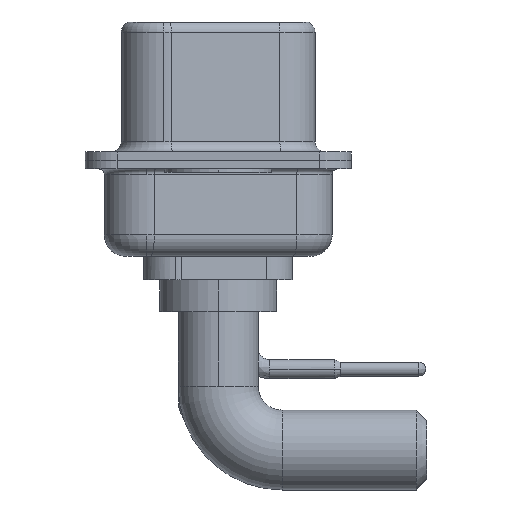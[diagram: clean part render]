
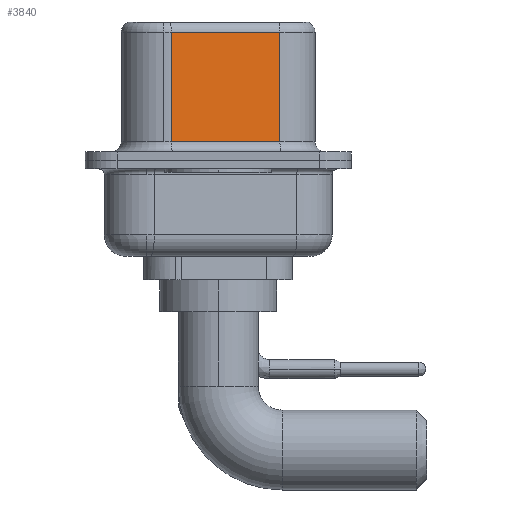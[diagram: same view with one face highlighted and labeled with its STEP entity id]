
A CAD part, left-side view. The second image highlights one B-rep face of the part: STEP entity #3840.
In plain terms, the highlighted planar face has unit normal (-0.985, -0.174, 0).
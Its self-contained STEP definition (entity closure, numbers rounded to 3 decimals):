
#580 = FACE_OUTER_BOUND ( 'NONE', #864, .T. ) ;
#864 = EDGE_LOOP ( 'NONE', ( #958, #6412, #3477, #17819 ) ) ;
#927 = EDGE_CURVE ( 'NONE', #14997, #15901, #13058, .T. ) ;
#958 = ORIENTED_EDGE ( 'NONE', *, *, #11378, .F. ) ;
#1845 = CARTESIAN_POINT ( 'NONE',  ( 4.555, -2.897, 0.9 ) ) ;
#2016 = DIRECTION ( 'NONE',  ( 0.985, 0.174, 0. ) ) ;
#2965 = CARTESIAN_POINT ( 'NONE',  ( 3.655, 2.203, 0.9 ) ) ;
#3426 = VECTOR ( 'NONE', #6063, 1000. ) ;
#3477 = ORIENTED_EDGE ( 'NONE', *, *, #8779, .T. ) ;
#3755 = DIRECTION ( 'NONE',  ( -0.174, 0.985, 0. ) ) ;
#3840 = ADVANCED_FACE ( 'NONE', ( #580 ), #7730, .F. ) ;
#4393 = VECTOR ( 'NONE', #17461, 1000. ) ;
#4451 = VECTOR ( 'NONE', #6938, 1000. ) ;
#4848 = VERTEX_POINT ( 'NONE', #15828 ) ;
#6063 = DIRECTION ( 'NONE',  ( 0., 0., -1. ) ) ;
#6412 = ORIENTED_EDGE ( 'NONE', *, *, #9795, .T. ) ;
#6938 = DIRECTION ( 'NONE',  ( 0.174, -0.985, 0. ) ) ;
#7673 = DIRECTION ( 'NONE',  ( -0.174, 0.985, 0. ) ) ;
#7730 = PLANE ( 'NONE',  #13802 ) ;
#7784 = CARTESIAN_POINT ( 'NONE',  ( 3.655, 2.203, 6.52 ) ) ;
#8779 = EDGE_CURVE ( 'NONE', #17406, #14997, #15244, .T. ) ;
#9795 = EDGE_CURVE ( 'NONE', #4848, #17406, #15038, .T. ) ;
#11378 = EDGE_CURVE ( 'NONE', #4848, #15901, #17837, .T. ) ;
#13058 = LINE ( 'NONE', #13146, #4451 ) ;
#13146 = CARTESIAN_POINT ( 'NONE',  ( 4.555, -2.897, 0.9 ) ) ;
#13497 = CARTESIAN_POINT ( 'NONE',  ( 4.555, -2.897, 6.02 ) ) ;
#13802 = AXIS2_PLACEMENT_3D ( 'NONE', #15384, #2016, #3755 ) ;
#14242 = VECTOR ( 'NONE', #7673, 1000. ) ;
#14997 = VERTEX_POINT ( 'NONE', #2965 ) ;
#15038 = LINE ( 'NONE', #13497, #14242 ) ;
#15244 = LINE ( 'NONE', #7784, #3426 ) ;
#15384 = CARTESIAN_POINT ( 'NONE',  ( 4.555, -2.897, 6.52 ) ) ;
#15505 = CARTESIAN_POINT ( 'NONE',  ( 3.655, 2.203, 6.02 ) ) ;
#15828 = CARTESIAN_POINT ( 'NONE',  ( 4.555, -2.897, 6.02 ) ) ;
#15901 = VERTEX_POINT ( 'NONE', #1845 ) ;
#17406 = VERTEX_POINT ( 'NONE', #15505 ) ;
#17461 = DIRECTION ( 'NONE',  ( 0., 0., -1. ) ) ;
#17819 = ORIENTED_EDGE ( 'NONE', *, *, #927, .T. ) ;
#17837 = LINE ( 'NONE', #18921, #4393 ) ;
#18921 = CARTESIAN_POINT ( 'NONE',  ( 4.555, -2.897, 6.52 ) ) ;
